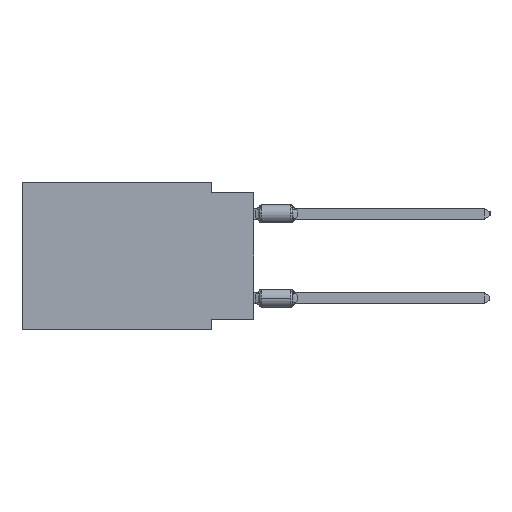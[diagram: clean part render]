
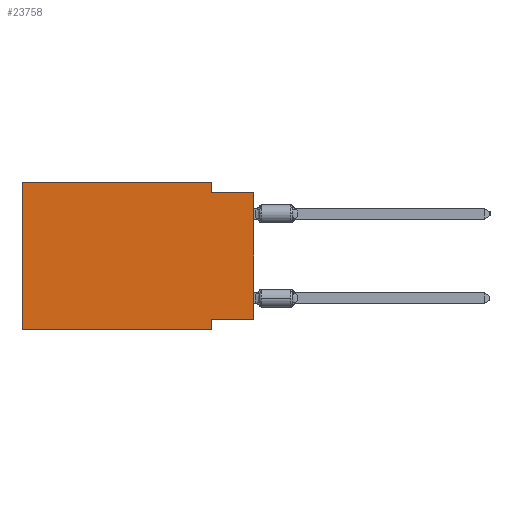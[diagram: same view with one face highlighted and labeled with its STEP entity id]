
A CAD part, left-side view. The second image highlights one B-rep face of the part: STEP entity #23758.
In plain terms, the highlighted planar face has unit normal (-1, 0, 0).
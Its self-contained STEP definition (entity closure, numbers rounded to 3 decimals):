
#415 = DIRECTION ( 'NONE',  ( 0., -1., 0. ) ) ;
#1023 = DIRECTION ( 'NONE',  ( 0., 0., 1. ) ) ;
#1377 = CARTESIAN_POINT ( 'NONE',  ( 0., 0., -0.635 ) ) ;
#3029 = ORIENTED_EDGE ( 'NONE', *, *, #21738, .T. ) ;
#3060 = VERTEX_POINT ( 'NONE', #30220 ) ;
#3286 = LINE ( 'NONE', #48678, #8329 ) ;
#3444 = DIRECTION ( 'NONE',  ( 0., 0., -1. ) ) ;
#4163 = ORIENTED_EDGE ( 'NONE', *, *, #11311, .T. ) ;
#4455 = CARTESIAN_POINT ( 'NONE',  ( 0., 0., -8.255 ) ) ;
#4720 = CARTESIAN_POINT ( 'NONE',  ( 0., 2.54, 0. ) ) ;
#5459 = VERTEX_POINT ( 'NONE', #11871 ) ;
#5974 = VECTOR ( 'NONE', #46361, 1000. ) ;
#6436 = ORIENTED_EDGE ( 'NONE', *, *, #11444, .F. ) ;
#6545 = CARTESIAN_POINT ( 'NONE',  ( 0., 0., 0. ) ) ;
#6981 = ORIENTED_EDGE ( 'NONE', *, *, #15636, .F. ) ;
#8329 = VECTOR ( 'NONE', #18425, 1000. ) ;
#8504 = CARTESIAN_POINT ( 'NONE',  ( 0., 13.97, -8.89 ) ) ;
#9306 = VERTEX_POINT ( 'NONE', #4720 ) ;
#11142 = FACE_OUTER_BOUND ( 'NONE', #32129, .T. ) ;
#11311 = EDGE_CURVE ( 'NONE', #48352, #39427, #19261, .T. ) ;
#11444 = EDGE_CURVE ( 'NONE', #9306, #3060, #47493, .T. ) ;
#11802 = CARTESIAN_POINT ( 'NONE',  ( 0., 0., -8.255 ) ) ;
#11871 = CARTESIAN_POINT ( 'NONE',  ( 0., 0., -0.635 ) ) ;
#12873 = CARTESIAN_POINT ( 'NONE',  ( 0., 2.54, -8.89 ) ) ;
#12939 = LINE ( 'NONE', #31768, #43203 ) ;
#14738 = DIRECTION ( 'NONE',  ( 0., 0., 1. ) ) ;
#15636 = EDGE_CURVE ( 'NONE', #36812, #39427, #3286, .T. ) ;
#18425 = DIRECTION ( 'NONE',  ( 0., 0., -1. ) ) ;
#19001 = LINE ( 'NONE', #1377, #26603 ) ;
#19261 = LINE ( 'NONE', #34385, #40522 ) ;
#21462 = ORIENTED_EDGE ( 'NONE', *, *, #36709, .F. ) ;
#21738 = EDGE_CURVE ( 'NONE', #30864, #5459, #30074, .T. ) ;
#22294 = CARTESIAN_POINT ( 'NONE',  ( 0., 13.97, 0. ) ) ;
#22312 = ORIENTED_EDGE ( 'NONE', *, *, #46307, .F. ) ;
#22545 = DIRECTION ( 'NONE',  ( 1., 0., 0. ) ) ;
#23562 = EDGE_CURVE ( 'NONE', #24851, #9306, #24798, .T. ) ;
#23758 = ADVANCED_FACE ( 'NONE', ( #11142 ), #41384, .F. ) ;
#24431 = DIRECTION ( 'NONE',  ( 0., -1., 0. ) ) ;
#24798 = LINE ( 'NONE', #39195, #39165 ) ;
#24851 = VERTEX_POINT ( 'NONE', #44864 ) ;
#26603 = VECTOR ( 'NONE', #24431, 1000. ) ;
#28130 = AXIS2_PLACEMENT_3D ( 'NONE', #22294, #22545, #3444 ) ;
#28660 = VECTOR ( 'NONE', #34013, 1000. ) ;
#30074 = LINE ( 'NONE', #6545, #36023 ) ;
#30220 = CARTESIAN_POINT ( 'NONE',  ( 0., 2.54, -0.635 ) ) ;
#30864 = VERTEX_POINT ( 'NONE', #11802 ) ;
#30979 = LINE ( 'NONE', #4455, #5974 ) ;
#31136 = CARTESIAN_POINT ( 'NONE',  ( 0., 2.54, -8.255 ) ) ;
#31768 = CARTESIAN_POINT ( 'NONE',  ( 0., 13.97, 0. ) ) ;
#32129 = EDGE_LOOP ( 'NONE', ( #3029, #21462, #6436, #45408, #43463, #4163, #6981, #22312 ) ) ;
#34013 = DIRECTION ( 'NONE',  ( 0., 0., -1. ) ) ;
#34385 = CARTESIAN_POINT ( 'NONE',  ( 0., 13.97, -8.89 ) ) ;
#36023 = VECTOR ( 'NONE', #14738, 1000. ) ;
#36709 = EDGE_CURVE ( 'NONE', #3060, #5459, #19001, .T. ) ;
#36812 = VERTEX_POINT ( 'NONE', #31136 ) ;
#39165 = VECTOR ( 'NONE', #39440, 1000. ) ;
#39195 = CARTESIAN_POINT ( 'NONE',  ( 0., 13.97, 0. ) ) ;
#39427 = VERTEX_POINT ( 'NONE', #12873 ) ;
#39440 = DIRECTION ( 'NONE',  ( 0., -1., 0. ) ) ;
#40522 = VECTOR ( 'NONE', #415, 1000. ) ;
#41384 = PLANE ( 'NONE',  #28130 ) ;
#42824 = EDGE_CURVE ( 'NONE', #48352, #24851, #12939, .T. ) ;
#43203 = VECTOR ( 'NONE', #1023, 1000. ) ;
#43463 = ORIENTED_EDGE ( 'NONE', *, *, #42824, .F. ) ;
#44023 = CARTESIAN_POINT ( 'NONE',  ( 0., 2.54, 0. ) ) ;
#44864 = CARTESIAN_POINT ( 'NONE',  ( 0., 13.97, 0. ) ) ;
#45408 = ORIENTED_EDGE ( 'NONE', *, *, #23562, .F. ) ;
#46307 = EDGE_CURVE ( 'NONE', #30864, #36812, #30979, .T. ) ;
#46361 = DIRECTION ( 'NONE',  ( 0., 1., 0. ) ) ;
#47493 = LINE ( 'NONE', #44023, #28660 ) ;
#48352 = VERTEX_POINT ( 'NONE', #8504 ) ;
#48678 = CARTESIAN_POINT ( 'NONE',  ( 0., 2.54, -8.89 ) ) ;
